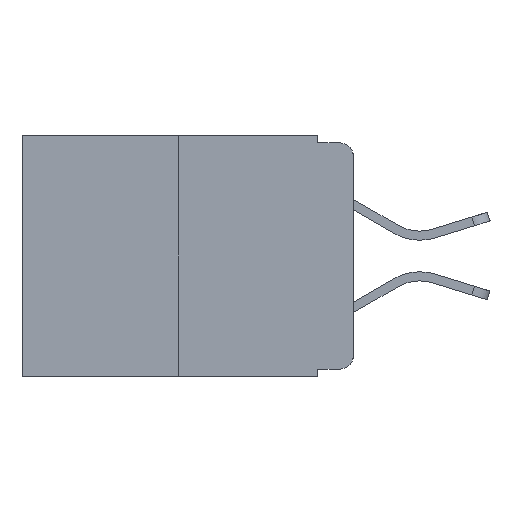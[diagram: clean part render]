
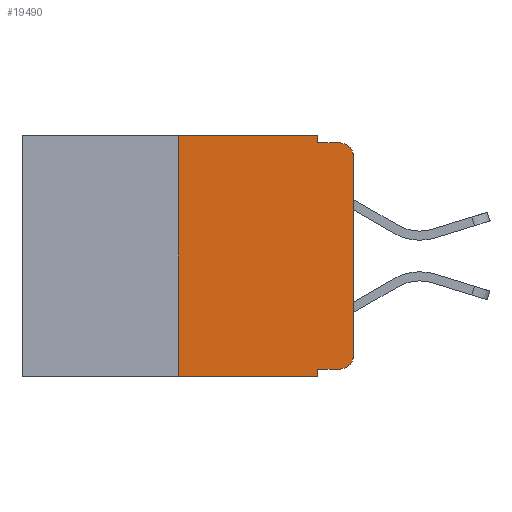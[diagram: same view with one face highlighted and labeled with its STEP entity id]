
A CAD part, left-side view. The second image highlights one B-rep face of the part: STEP entity #19490.
In plain terms, the highlighted planar face has unit normal (-1, 0, 0).
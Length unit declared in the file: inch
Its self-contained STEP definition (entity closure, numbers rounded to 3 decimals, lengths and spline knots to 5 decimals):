
#113 = VECTOR ( 'NONE', #12250, 39.37008 ) ;
#233 = CARTESIAN_POINT ( 'NONE',  ( 0., 0.051, -0.01 ) ) ;
#989 = ORIENTED_EDGE ( 'NONE', *, *, #9501, .F. ) ;
#997 = VERTEX_POINT ( 'NONE', #22717 ) ;
#1522 = LINE ( 'NONE', #18592, #7401 ) ;
#2516 = CARTESIAN_POINT ( 'NONE',  ( 0., 0., -0.03 ) ) ;
#2706 = VERTEX_POINT ( 'NONE', #11335 ) ;
#2774 = LINE ( 'NONE', #20297, #14185 ) ;
#2963 = ORIENTED_EDGE ( 'NONE', *, *, #8058, .F. ) ;
#3001 = ORIENTED_EDGE ( 'NONE', *, *, #14043, .T. ) ;
#3088 = DIRECTION ( 'NONE',  ( 0., 0., 1. ) ) ;
#3638 = EDGE_CURVE ( 'NONE', #8941, #8982, #1522, .T. ) ;
#4078 = ORIENTED_EDGE ( 'NONE', *, *, #19102, .T. ) ;
#4824 = ORIENTED_EDGE ( 'NONE', *, *, #3638, .F. ) ;
#5078 = VERTEX_POINT ( 'NONE', #26876 ) ;
#5333 = CARTESIAN_POINT ( 'NONE',  ( 0., 0.25, 0. ) ) ;
#6484 = ORIENTED_EDGE ( 'NONE', *, *, #13895, .F. ) ;
#6845 = ORIENTED_EDGE ( 'NONE', *, *, #15073, .T. ) ;
#6904 = CARTESIAN_POINT ( 'NONE',  ( 0., 0.051, -0.333 ) ) ;
#7022 = PLANE ( 'NONE',  #8233 ) ;
#7401 = VECTOR ( 'NONE', #8332, 39.37008 ) ;
#7978 = DIRECTION ( 'NONE',  ( 0., 0., 1. ) ) ;
#8058 = EDGE_CURVE ( 'NONE', #20605, #11750, #10547, .T. ) ;
#8188 = VERTEX_POINT ( 'NONE', #20299 ) ;
#8233 = AXIS2_PLACEMENT_3D ( 'NONE', #9197, #11313, #25523 ) ;
#8332 = DIRECTION ( 'NONE',  ( 0., 0., -1. ) ) ;
#8790 = VECTOR ( 'NONE', #18443, 39.37008 ) ;
#8941 = VERTEX_POINT ( 'NONE', #10061 ) ;
#8982 = VERTEX_POINT ( 'NONE', #22409 ) ;
#9197 = CARTESIAN_POINT ( 'NONE',  ( 0., 0.473, 0. ) ) ;
#9501 = EDGE_CURVE ( 'NONE', #5078, #997, #17184, .T. ) ;
#9986 = CARTESIAN_POINT ( 'NONE',  ( 0., 0.02, -0.03 ) ) ;
#10061 = CARTESIAN_POINT ( 'NONE',  ( 0., 0.051, -0.333 ) ) ;
#10123 = CARTESIAN_POINT ( 'NONE',  ( 0., 0.051, 0. ) ) ;
#10547 = LINE ( 'NONE', #5333, #15413 ) ;
#11313 = DIRECTION ( 'NONE',  ( 1., 0., 0. ) ) ;
#11335 = CARTESIAN_POINT ( 'NONE',  ( 0., 0.02, -0.333 ) ) ;
#11750 = VERTEX_POINT ( 'NONE', #25428 ) ;
#12113 = DIRECTION ( 'NONE',  ( 0., 0., -1. ) ) ;
#12250 = DIRECTION ( 'NONE',  ( 0., 0., -1. ) ) ;
#12763 = DIRECTION ( 'NONE',  ( -1., 0., 0. ) ) ;
#13709 = EDGE_CURVE ( 'NONE', #997, #8188, #16598, .T. ) ;
#13895 = EDGE_CURVE ( 'NONE', #11750, #5078, #18143, .T. ) ;
#14043 = EDGE_CURVE ( 'NONE', #20605, #8982, #19068, .T. ) ;
#14185 = VECTOR ( 'NONE', #7978, 39.37008 ) ;
#15073 = EDGE_CURVE ( 'NONE', #23126, #8188, #21189, .T. ) ;
#15374 = DIRECTION ( 'NONE',  ( 0., -1., 0. ) ) ;
#15413 = VECTOR ( 'NONE', #3088, 39.37008 ) ;
#15469 = VERTEX_POINT ( 'NONE', #25468 ) ;
#16135 = AXIS2_PLACEMENT_3D ( 'NONE', #24871, #12763, #26946 ) ;
#16425 = CARTESIAN_POINT ( 'NONE',  ( 0., 0.473, -0.343 ) ) ;
#16598 = LINE ( 'NONE', #233, #26719 ) ;
#16805 = EDGE_LOOP ( 'NONE', ( #4078, #6845, #27010, #989, #6484, #2963, #3001, #4824, #27073, #20788 ) ) ;
#16931 = CIRCLE ( 'NONE', #16135, 0.02 ) ;
#17184 = LINE ( 'NONE', #10123, #113 ) ;
#17525 = VECTOR ( 'NONE', #21929, 39.37008 ) ;
#18143 = LINE ( 'NONE', #19926, #17525 ) ;
#18443 = DIRECTION ( 'NONE',  ( 0., -1., 0. ) ) ;
#18592 = CARTESIAN_POINT ( 'NONE',  ( 0., 0.051, 0. ) ) ;
#18620 = VECTOR ( 'NONE', #15374, 39.37008 ) ;
#19068 = LINE ( 'NONE', #16425, #8790 ) ;
#19102 = EDGE_CURVE ( 'NONE', #15469, #23126, #2774, .T. ) ;
#19255 = LINE ( 'NONE', #6904, #18620 ) ;
#19334 = DIRECTION ( 'NONE',  ( 0., -1., 0. ) ) ;
#19490 = ADVANCED_FACE ( 'NONE', ( #26839 ), #7022, .F. ) ;
#19926 = CARTESIAN_POINT ( 'NONE',  ( 0., 0.473, 0. ) ) ;
#20297 = CARTESIAN_POINT ( 'NONE',  ( 0., 0., 0. ) ) ;
#20299 = CARTESIAN_POINT ( 'NONE',  ( 0., 0.02, -0.01 ) ) ;
#20605 = VERTEX_POINT ( 'NONE', #21064 ) ;
#20788 = ORIENTED_EDGE ( 'NONE', *, *, #22273, .T. ) ;
#21064 = CARTESIAN_POINT ( 'NONE',  ( 0., 0.25, -0.343 ) ) ;
#21189 = CIRCLE ( 'NONE', #24618, 0.02 ) ;
#21929 = DIRECTION ( 'NONE',  ( 0., -1., 0. ) ) ;
#22273 = EDGE_CURVE ( 'NONE', #2706, #15469, #16931, .T. ) ;
#22409 = CARTESIAN_POINT ( 'NONE',  ( 0., 0.051, -0.343 ) ) ;
#22717 = CARTESIAN_POINT ( 'NONE',  ( 0., 0.051, -0.01 ) ) ;
#23126 = VERTEX_POINT ( 'NONE', #2516 ) ;
#24216 = DIRECTION ( 'NONE',  ( -1., 0., 0. ) ) ;
#24618 = AXIS2_PLACEMENT_3D ( 'NONE', #9986, #24216, #12113 ) ;
#24871 = CARTESIAN_POINT ( 'NONE',  ( 0., 0.02, -0.313 ) ) ;
#25428 = CARTESIAN_POINT ( 'NONE',  ( 0., 0.25, 0. ) ) ;
#25468 = CARTESIAN_POINT ( 'NONE',  ( 0., 0., -0.313 ) ) ;
#25523 = DIRECTION ( 'NONE',  ( 0., 0., -1. ) ) ;
#26414 = EDGE_CURVE ( 'NONE', #8941, #2706, #19255, .T. ) ;
#26719 = VECTOR ( 'NONE', #19334, 39.37008 ) ;
#26839 = FACE_OUTER_BOUND ( 'NONE', #16805, .T. ) ;
#26876 = CARTESIAN_POINT ( 'NONE',  ( 0., 0.051, 0. ) ) ;
#26946 = DIRECTION ( 'NONE',  ( 0., 0., -1. ) ) ;
#27010 = ORIENTED_EDGE ( 'NONE', *, *, #13709, .F. ) ;
#27073 = ORIENTED_EDGE ( 'NONE', *, *, #26414, .T. ) ;
